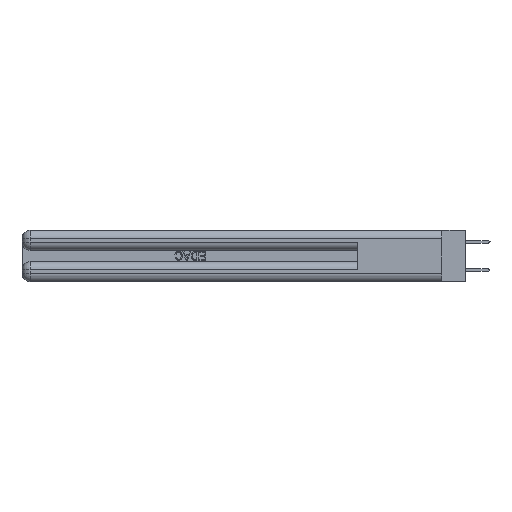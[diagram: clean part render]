
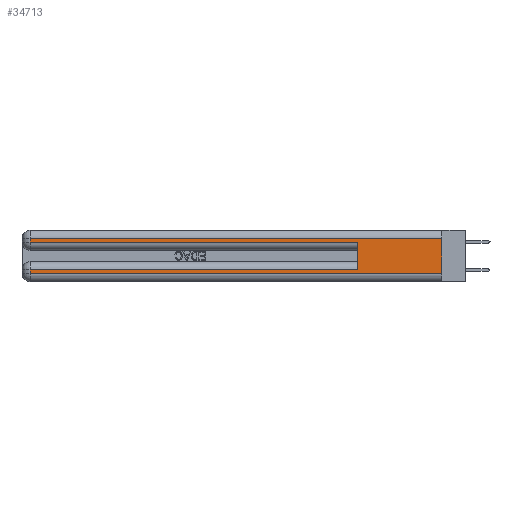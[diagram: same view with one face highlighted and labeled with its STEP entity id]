
A CAD part, left-side view. The second image highlights one B-rep face of the part: STEP entity #34713.
In plain terms, the highlighted planar face has unit normal (-1, 0, 0).
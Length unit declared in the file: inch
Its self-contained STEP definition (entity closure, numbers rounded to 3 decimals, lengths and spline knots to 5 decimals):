
#703 = EDGE_CURVE ( 'NONE', #38931, #23110, #42296, .T. ) ;
#764 = VERTEX_POINT ( 'NONE', #28747 ) ;
#1415 = CARTESIAN_POINT ( 'NONE',  ( 0., 0., 0.37 ) ) ;
#1666 = EDGE_CURVE ( 'NONE', #764, #39778, #20901, .T. ) ;
#1998 = AXIS2_PLACEMENT_3D ( 'NONE', #1415, #4667, #30677 ) ;
#4667 = DIRECTION ( 'NONE',  ( 1., 0., 0. ) ) ;
#4722 = ORIENTED_EDGE ( 'NONE', *, *, #22941, .T. ) ;
#9143 = LINE ( 'NONE', #13990, #29255 ) ;
#10348 = VECTOR ( 'NONE', #25531, 39.37008 ) ;
#10976 = EDGE_CURVE ( 'NONE', #38931, #28246, #37226, .T. ) ;
#13667 = DIRECTION ( 'NONE',  ( 0., 0., -1. ) ) ;
#13877 = ORIENTED_EDGE ( 'NONE', *, *, #10976, .T. ) ;
#13990 = CARTESIAN_POINT ( 'NONE',  ( 0., 2.94, 0.37 ) ) ;
#14053 = CARTESIAN_POINT ( 'NONE',  ( 0., 0., 0.06 ) ) ;
#14658 = CARTESIAN_POINT ( 'NONE',  ( 0., 2.94, 0.31 ) ) ;
#14782 = DIRECTION ( 'NONE',  ( 0., 0., -1. ) ) ;
#15499 = VERTEX_POINT ( 'NONE', #45365 ) ;
#15673 = DIRECTION ( 'NONE',  ( 0., 0., 1. ) ) ;
#16199 = PLANE ( 'NONE',  #1998 ) ;
#16686 = CARTESIAN_POINT ( 'NONE',  ( 0., 2.94, 0.285 ) ) ;
#18241 = VECTOR ( 'NONE', #44967, 39.37008 ) ;
#18307 = LINE ( 'NONE', #26796, #44147 ) ;
#18827 = CARTESIAN_POINT ( 'NONE',  ( 0., 2.94, 0.06 ) ) ;
#20132 = LINE ( 'NONE', #21844, #10348 ) ;
#20901 = LINE ( 'NONE', #25909, #45532 ) ;
#21844 = CARTESIAN_POINT ( 'NONE',  ( 0., 0., 0.285 ) ) ;
#21949 = FACE_OUTER_BOUND ( 'NONE', #43152, .T. ) ;
#22291 = LINE ( 'NONE', #14053, #29743 ) ;
#22941 = EDGE_CURVE ( 'NONE', #39778, #23110, #22291, .T. ) ;
#23110 = VERTEX_POINT ( 'NONE', #40820 ) ;
#24517 = VECTOR ( 'NONE', #42848, 39.37008 ) ;
#25006 = DIRECTION ( 'NONE',  ( 0., -1., 0. ) ) ;
#25531 = DIRECTION ( 'NONE',  ( 0., -1., 0. ) ) ;
#25859 = LINE ( 'NONE', #39653, #38457 ) ;
#25909 = CARTESIAN_POINT ( 'NONE',  ( 0., 2.94, 0.37 ) ) ;
#26607 = VERTEX_POINT ( 'NONE', #16686 ) ;
#26796 = CARTESIAN_POINT ( 'NONE',  ( 0., 0.6, 0.145 ) ) ;
#27959 = CARTESIAN_POINT ( 'NONE',  ( 0., 0., 0.37 ) ) ;
#28246 = VERTEX_POINT ( 'NONE', #14658 ) ;
#28747 = CARTESIAN_POINT ( 'NONE',  ( 0., 2.94, 0.085 ) ) ;
#28877 = VERTEX_POINT ( 'NONE', #29635 ) ;
#29255 = VECTOR ( 'NONE', #13667, 39.37008 ) ;
#29635 = CARTESIAN_POINT ( 'NONE',  ( 0., 0.6, 0.085 ) ) ;
#29743 = VECTOR ( 'NONE', #25006, 39.37008 ) ;
#29784 = ORIENTED_EDGE ( 'NONE', *, *, #1666, .T. ) ;
#30677 = DIRECTION ( 'NONE',  ( 0., 0., -1. ) ) ;
#31397 = ORIENTED_EDGE ( 'NONE', *, *, #35852, .T. ) ;
#32358 = EDGE_CURVE ( 'NONE', #28246, #26607, #9143, .T. ) ;
#33601 = CARTESIAN_POINT ( 'NONE',  ( 0., 0., 0.31 ) ) ;
#34713 = ADVANCED_FACE ( 'NONE', ( #21949 ), #16199, .F. ) ;
#34803 = ORIENTED_EDGE ( 'NONE', *, *, #703, .F. ) ;
#35852 = EDGE_CURVE ( 'NONE', #28877, #764, #25859, .T. ) ;
#36154 = EDGE_CURVE ( 'NONE', #28877, #15499, #18307, .T. ) ;
#37226 = LINE ( 'NONE', #33601, #18241 ) ;
#38457 = VECTOR ( 'NONE', #43326, 39.37008 ) ;
#38931 = VERTEX_POINT ( 'NONE', #39152 ) ;
#39152 = CARTESIAN_POINT ( 'NONE',  ( 0., 0., 0.31 ) ) ;
#39653 = CARTESIAN_POINT ( 'NONE',  ( 0., 0., 0.085 ) ) ;
#39778 = VERTEX_POINT ( 'NONE', #18827 ) ;
#40237 = ORIENTED_EDGE ( 'NONE', *, *, #36154, .F. ) ;
#40820 = CARTESIAN_POINT ( 'NONE',  ( 0., 0., 0.06 ) ) ;
#40966 = EDGE_CURVE ( 'NONE', #26607, #15499, #20132, .T. ) ;
#42296 = LINE ( 'NONE', #27959, #24517 ) ;
#42848 = DIRECTION ( 'NONE',  ( 0., 0., -1. ) ) ;
#43152 = EDGE_LOOP ( 'NONE', ( #34803, #13877, #47326, #46625, #40237, #31397, #29784, #4722 ) ) ;
#43326 = DIRECTION ( 'NONE',  ( 0., 1., 0. ) ) ;
#44147 = VECTOR ( 'NONE', #15673, 39.37008 ) ;
#44967 = DIRECTION ( 'NONE',  ( 0., 1., 0. ) ) ;
#45365 = CARTESIAN_POINT ( 'NONE',  ( 0., 0.6, 0.285 ) ) ;
#45532 = VECTOR ( 'NONE', #14782, 39.37008 ) ;
#46625 = ORIENTED_EDGE ( 'NONE', *, *, #40966, .T. ) ;
#47326 = ORIENTED_EDGE ( 'NONE', *, *, #32358, .T. ) ;
